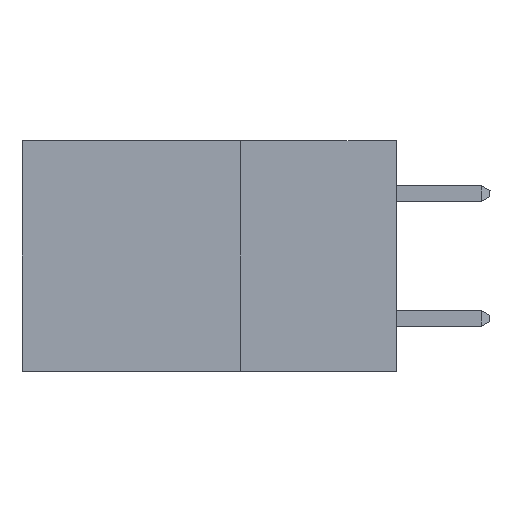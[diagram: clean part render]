
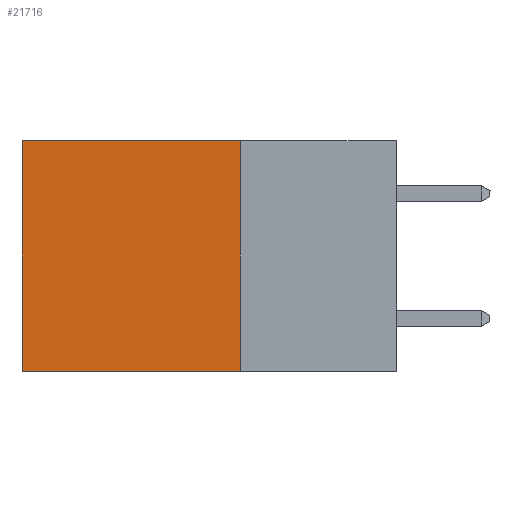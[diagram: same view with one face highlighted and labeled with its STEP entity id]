
A CAD part, left-side view. The second image highlights one B-rep face of the part: STEP entity #21716.
In plain terms, the highlighted planar face has unit normal (-1, 0, 0).
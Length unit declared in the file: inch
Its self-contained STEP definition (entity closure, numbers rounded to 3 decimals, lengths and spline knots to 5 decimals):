
#83 = LINE ( 'NONE', #3404, #18276 ) ;
#636 = DIRECTION ( 'NONE',  ( 0., 0., -1. ) ) ;
#909 = CARTESIAN_POINT ( 'NONE',  ( 0.298, 0.25, -0.37 ) ) ;
#933 = CARTESIAN_POINT ( 'NONE',  ( 0.298, 0.25, 0. ) ) ;
#1288 = DIRECTION ( 'NONE',  ( 0., 0., -1. ) ) ;
#2427 = EDGE_CURVE ( 'NONE', #10852, #19557, #83, .T. ) ;
#2889 = VERTEX_POINT ( 'NONE', #21202 ) ;
#3404 = CARTESIAN_POINT ( 'NONE',  ( 0.298, 0.25, 0. ) ) ;
#4739 = DIRECTION ( 'NONE',  ( 0., 0., -1. ) ) ;
#7960 = ORIENTED_EDGE ( 'NONE', *, *, #2427, .F. ) ;
#9172 = DIRECTION ( 'NONE',  ( 0., 1., 0. ) ) ;
#10174 = CARTESIAN_POINT ( 'NONE',  ( 0.298, 0.6, -0.37 ) ) ;
#10852 = VERTEX_POINT ( 'NONE', #933 ) ;
#10859 = DIRECTION ( 'NONE',  ( 0., 1., 0. ) ) ;
#10949 = EDGE_CURVE ( 'NONE', #10852, #2889, #22079, .T. ) ;
#13597 = CARTESIAN_POINT ( 'NONE',  ( 0.298, 0.25, 0. ) ) ;
#14787 = LINE ( 'NONE', #17067, #28538 ) ;
#14829 = ORIENTED_EDGE ( 'NONE', *, *, #10949, .T. ) ;
#15250 = VECTOR ( 'NONE', #10859, 39.37008 ) ;
#16106 = DIRECTION ( 'NONE',  ( 1., 0., 0. ) ) ;
#16451 = VERTEX_POINT ( 'NONE', #10174 ) ;
#17067 = CARTESIAN_POINT ( 'NONE',  ( 0.298, 0.6, 0. ) ) ;
#18201 = EDGE_CURVE ( 'NONE', #19557, #16451, #27456, .T. ) ;
#18242 = CARTESIAN_POINT ( 'NONE',  ( 0.298, 0.25, -0.37 ) ) ;
#18276 = VECTOR ( 'NONE', #636, 39.37008 ) ;
#19557 = VERTEX_POINT ( 'NONE', #18242 ) ;
#21175 = EDGE_LOOP ( 'NONE', ( #27514, #24356, #7960, #14829 ) ) ;
#21202 = CARTESIAN_POINT ( 'NONE',  ( 0.298, 0.6, 0. ) ) ;
#21716 = ADVANCED_FACE ( 'NONE', ( #30149 ), #28240, .F. ) ;
#22079 = LINE ( 'NONE', #26281, #26996 ) ;
#24356 = ORIENTED_EDGE ( 'NONE', *, *, #18201, .F. ) ;
#26281 = CARTESIAN_POINT ( 'NONE',  ( 0.298, 0.25, 0. ) ) ;
#26996 = VECTOR ( 'NONE', #9172, 39.37008 ) ;
#27321 = EDGE_CURVE ( 'NONE', #2889, #16451, #14787, .T. ) ;
#27456 = LINE ( 'NONE', #909, #15250 ) ;
#27514 = ORIENTED_EDGE ( 'NONE', *, *, #27321, .T. ) ;
#28240 = PLANE ( 'NONE',  #28661 ) ;
#28538 = VECTOR ( 'NONE', #4739, 39.37008 ) ;
#28661 = AXIS2_PLACEMENT_3D ( 'NONE', #13597, #16106, #1288 ) ;
#30149 = FACE_OUTER_BOUND ( 'NONE', #21175, .T. ) ;
